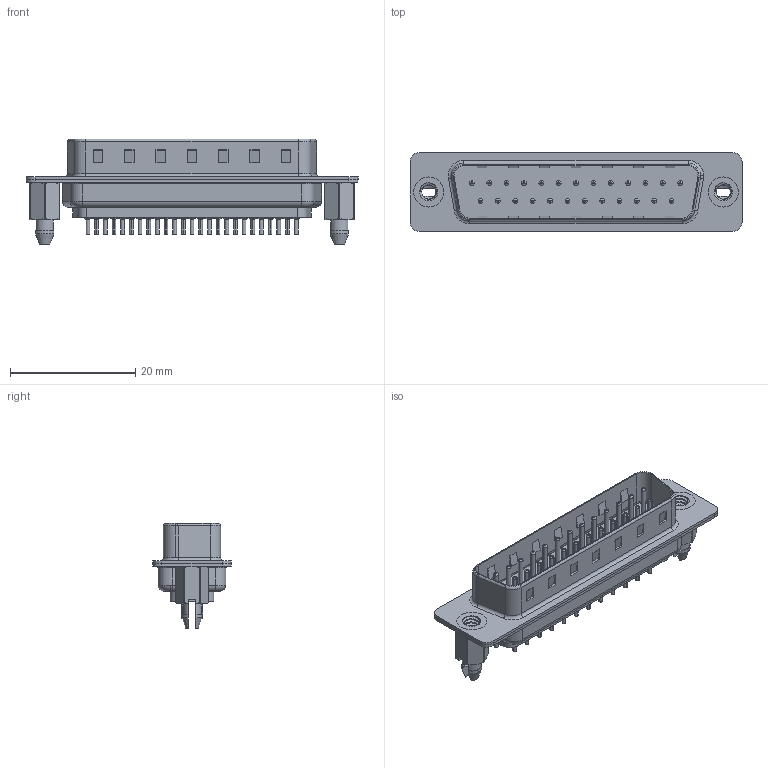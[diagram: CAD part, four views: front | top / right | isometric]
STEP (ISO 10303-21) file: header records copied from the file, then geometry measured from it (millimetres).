
FILE_DESCRIPTION (( 'STEP AP203' ), '1' );
FILE_NAME ('627-025-320-546.STEP', '2018-10-05T04:40:10', ( '' ), ( '' ), 'SwSTEP 2.0', 'SolidWorks 2016', '' );
FILE_SCHEMA (( 'CONFIG_CONTROL_DESIGN' ));
Length unit declared in the file: millimetre
Products named in the file (7): 627 4-40 Threaded Boardlock_LP; 627-025-320-546; 627 Housing_25 LP; 627 Shell Front_25 Contacts; 627 Shell Rear_25 Contacts; 627 Contact Row 1_20L; 627 Contact Row 2_20L
Assembly tree (30 placements, depth 2):
  627-025-320-546
    627 Housing_25 LP
    627 Shell Front_25 Contacts
    627 Shell Rear_25 Contacts
    627 Contact Row 1_20L  x13
    627 Contact Row 2_20L  x12
    627 4-40 Threaded Boardlock_LP  x2
Bounding box: 53 x 12.6 x 16.9 mm (x, y, z)
Volume: 2784.2 mm3; surface area: 7944.6 mm2
Topology: 30 solids, 30 shells, 2900 faces, 7616 edges, 4735 vertices
Faces by surface type: cylinder 1094, plane 803, torus 731, cone 266, bspline 6
Entity records: 26268 total; most frequent: CARTESIAN_POINT 5953, DIRECTION 4196, ORIENTED_EDGE 3826, EDGE_CURVE 1913, AXIS2_PLACEMENT_3D 1648, VERTEX_POINT 1223, EDGE_LOOP 910, LINE 900
